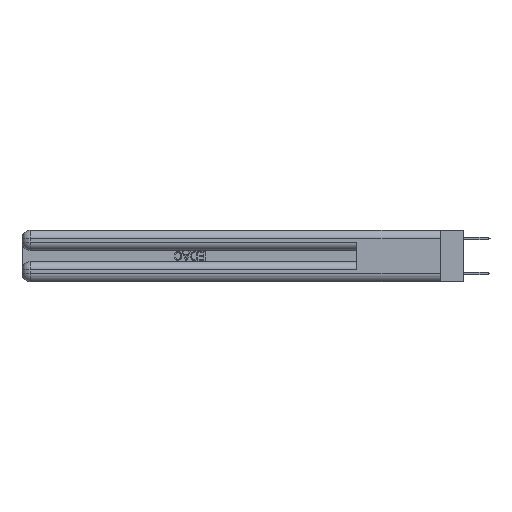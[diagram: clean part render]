
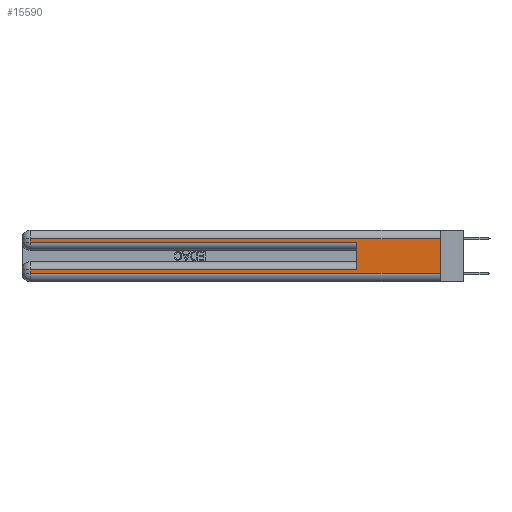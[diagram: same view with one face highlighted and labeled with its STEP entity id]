
A CAD part, left-side view. The second image highlights one B-rep face of the part: STEP entity #15590.
In plain terms, the highlighted planar face has unit normal (-1, 0, 0).
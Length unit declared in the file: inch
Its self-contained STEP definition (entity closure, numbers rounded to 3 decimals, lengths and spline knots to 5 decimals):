
#1641 = DIRECTION ( 'NONE',  ( 0., 0., -1. ) ) ;
#2133 = VERTEX_POINT ( 'NONE', #31432 ) ;
#3042 = LINE ( 'NONE', #5986, #28407 ) ;
#3128 = CARTESIAN_POINT ( 'NONE',  ( 0., 2.94, 0.285 ) ) ;
#3339 = VERTEX_POINT ( 'NONE', #28390 ) ;
#3349 = LINE ( 'NONE', #6953, #22430 ) ;
#3949 = CARTESIAN_POINT ( 'NONE',  ( 0., 0., 0.37 ) ) ;
#4199 = VERTEX_POINT ( 'NONE', #10196 ) ;
#4277 = VECTOR ( 'NONE', #10032, 39.37008 ) ;
#5363 = ORIENTED_EDGE ( 'NONE', *, *, #19591, .T. ) ;
#5393 = VECTOR ( 'NONE', #15787, 39.37008 ) ;
#5986 = CARTESIAN_POINT ( 'NONE',  ( 0., 0., 0.285 ) ) ;
#6134 = CARTESIAN_POINT ( 'NONE',  ( 0., 0., 0.37 ) ) ;
#6209 = LINE ( 'NONE', #13306, #5393 ) ;
#6899 = ORIENTED_EDGE ( 'NONE', *, *, #13360, .T. ) ;
#6953 = CARTESIAN_POINT ( 'NONE',  ( 0., 0., 0.085 ) ) ;
#8166 = VERTEX_POINT ( 'NONE', #20936 ) ;
#8334 = EDGE_CURVE ( 'NONE', #9360, #13028, #20479, .T. ) ;
#9360 = VERTEX_POINT ( 'NONE', #29861 ) ;
#9519 = DIRECTION ( 'NONE',  ( 0., 1., 0. ) ) ;
#10032 = DIRECTION ( 'NONE',  ( 0., 1., 0. ) ) ;
#10196 = CARTESIAN_POINT ( 'NONE',  ( 0., 0., 0.31 ) ) ;
#11289 = DIRECTION ( 'NONE',  ( 0., 0., -1. ) ) ;
#13028 = VERTEX_POINT ( 'NONE', #3128 ) ;
#13267 = VECTOR ( 'NONE', #1641, 39.37008 ) ;
#13306 = CARTESIAN_POINT ( 'NONE',  ( 0., 0.6, 0.145 ) ) ;
#13354 = ORIENTED_EDGE ( 'NONE', *, *, #18533, .T. ) ;
#13360 = EDGE_CURVE ( 'NONE', #8166, #3339, #3349, .T. ) ;
#13544 = VECTOR ( 'NONE', #26134, 39.37008 ) ;
#14392 = LINE ( 'NONE', #16936, #19315 ) ;
#15590 = ADVANCED_FACE ( 'NONE', ( #21904 ), #23368, .F. ) ;
#15787 = DIRECTION ( 'NONE',  ( 0., 0., 1. ) ) ;
#16936 = CARTESIAN_POINT ( 'NONE',  ( 0., 2.94, 0.37 ) ) ;
#17347 = DIRECTION ( 'NONE',  ( 0., -1., 0. ) ) ;
#18533 = EDGE_CURVE ( 'NONE', #2133, #19072, #26633, .T. ) ;
#18883 = ORIENTED_EDGE ( 'NONE', *, *, #30593, .T. ) ;
#19072 = VERTEX_POINT ( 'NONE', #21519 ) ;
#19315 = VECTOR ( 'NONE', #19354, 39.37008 ) ;
#19318 = EDGE_CURVE ( 'NONE', #4199, #9360, #24008, .T. ) ;
#19354 = DIRECTION ( 'NONE',  ( 0., 0., -1. ) ) ;
#19591 = EDGE_CURVE ( 'NONE', #13028, #29647, #3042, .T. ) ;
#19596 = VECTOR ( 'NONE', #17347, 39.37008 ) ;
#19904 = EDGE_LOOP ( 'NONE', ( #27832, #29699, #30237, #5363, #31015, #6899, #18883, #13354 ) ) ;
#19983 = AXIS2_PLACEMENT_3D ( 'NONE', #6134, #25750, #11289 ) ;
#20479 = LINE ( 'NONE', #31023, #13267 ) ;
#20879 = DIRECTION ( 'NONE',  ( 0., -1., 0. ) ) ;
#20936 = CARTESIAN_POINT ( 'NONE',  ( 0., 0.6, 0.085 ) ) ;
#21519 = CARTESIAN_POINT ( 'NONE',  ( 0., 0., 0.06 ) ) ;
#21904 = FACE_OUTER_BOUND ( 'NONE', #19904, .T. ) ;
#22342 = CARTESIAN_POINT ( 'NONE',  ( 0., 0., 0.31 ) ) ;
#22430 = VECTOR ( 'NONE', #9519, 39.37008 ) ;
#22841 = CARTESIAN_POINT ( 'NONE',  ( 0., 0.6, 0.285 ) ) ;
#23368 = PLANE ( 'NONE',  #19983 ) ;
#24008 = LINE ( 'NONE', #22342, #4277 ) ;
#24633 = EDGE_CURVE ( 'NONE', #4199, #19072, #26292, .T. ) ;
#25750 = DIRECTION ( 'NONE',  ( 1., 0., 0. ) ) ;
#26134 = DIRECTION ( 'NONE',  ( 0., 0., -1. ) ) ;
#26292 = LINE ( 'NONE', #3949, #13544 ) ;
#26633 = LINE ( 'NONE', #29177, #19596 ) ;
#27156 = EDGE_CURVE ( 'NONE', #8166, #29647, #6209, .T. ) ;
#27832 = ORIENTED_EDGE ( 'NONE', *, *, #24633, .F. ) ;
#28390 = CARTESIAN_POINT ( 'NONE',  ( 0., 2.94, 0.085 ) ) ;
#28407 = VECTOR ( 'NONE', #20879, 39.37008 ) ;
#29177 = CARTESIAN_POINT ( 'NONE',  ( 0., 0., 0.06 ) ) ;
#29647 = VERTEX_POINT ( 'NONE', #22841 ) ;
#29699 = ORIENTED_EDGE ( 'NONE', *, *, #19318, .T. ) ;
#29861 = CARTESIAN_POINT ( 'NONE',  ( 0., 2.94, 0.31 ) ) ;
#30237 = ORIENTED_EDGE ( 'NONE', *, *, #8334, .T. ) ;
#30593 = EDGE_CURVE ( 'NONE', #3339, #2133, #14392, .T. ) ;
#31015 = ORIENTED_EDGE ( 'NONE', *, *, #27156, .F. ) ;
#31023 = CARTESIAN_POINT ( 'NONE',  ( 0., 2.94, 0.37 ) ) ;
#31432 = CARTESIAN_POINT ( 'NONE',  ( 0., 2.94, 0.06 ) ) ;
